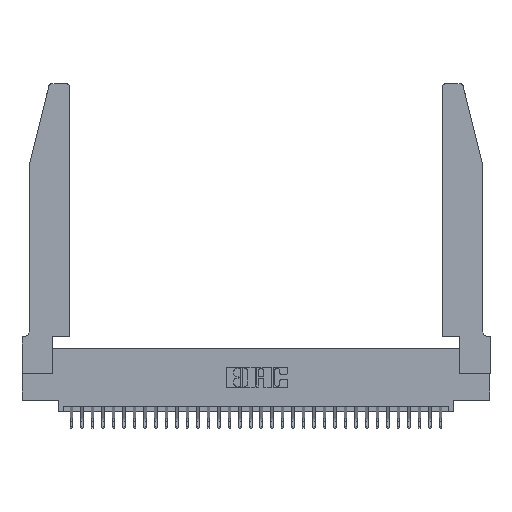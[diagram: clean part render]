
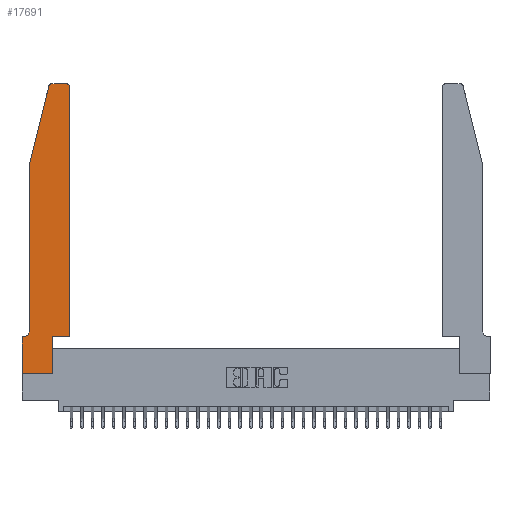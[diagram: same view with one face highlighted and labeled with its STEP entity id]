
A CAD part, top view. The second image highlights one B-rep face of the part: STEP entity #17691.
In plain terms, the highlighted planar face has unit normal (0, 0, 1).
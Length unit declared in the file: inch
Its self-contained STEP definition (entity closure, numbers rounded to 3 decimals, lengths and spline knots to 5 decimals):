
#825 = LINE ( 'NONE', #27042, #12400 ) ;
#1028 = ORIENTED_EDGE ( 'NONE', *, *, #27135, .T. ) ;
#1734 = CARTESIAN_POINT ( 'NONE',  ( 0., 0., 0.37 ) ) ;
#2498 = DIRECTION ( 'NONE',  ( 1., 0., 0. ) ) ;
#3057 = CARTESIAN_POINT ( 'NONE',  ( 0.0755, 2., 0.37 ) ) ;
#4718 = CARTESIAN_POINT ( 'NONE',  ( 0.284, 2.72, 0.37 ) ) ;
#4770 = CARTESIAN_POINT ( 'NONE',  ( 0.2865, 0.35, 0.37 ) ) ;
#4873 = CARTESIAN_POINT ( 'NONE',  ( 0.0755, 2., 0.37 ) ) ;
#4893 = VERTEX_POINT ( 'NONE', #19958 ) ;
#5174 = DIRECTION ( 'NONE',  ( -1., 0., 0. ) ) ;
#5564 = DIRECTION ( 'NONE',  ( 1., 0., 0. ) ) ;
#6221 = DIRECTION ( 'NONE',  ( 1., 0., 0. ) ) ;
#6347 = EDGE_CURVE ( 'NONE', #23144, #25207, #25120, .T. ) ;
#6566 = DIRECTION ( 'NONE',  ( 0., 0., -1. ) ) ;
#6980 = CARTESIAN_POINT ( 'NONE',  ( 0., 0., 0.37 ) ) ;
#7020 = VERTEX_POINT ( 'NONE', #27892 ) ;
#7575 = CIRCLE ( 'NONE', #29233, 0.03 ) ;
#7687 = EDGE_CURVE ( 'NONE', #19521, #7020, #26011, .T. ) ;
#7766 = CARTESIAN_POINT ( 'NONE',  ( 0.4505, 0.35, 0.37 ) ) ;
#8029 = PLANE ( 'NONE',  #14119 ) ;
#9557 = EDGE_CURVE ( 'NONE', #27238, #30307, #28830, .T. ) ;
#9586 = LINE ( 'NONE', #6980, #23934 ) ;
#9855 = CIRCLE ( 'NONE', #29030, 0.03 ) ;
#10363 = EDGE_LOOP ( 'NONE', ( #27302, #29611, #12300, #27228, #28320, #13306, #20744, #26653, #16598, #30921, #16795, #1028 ) ) ;
#11478 = CARTESIAN_POINT ( 'NONE',  ( 0., 0., 0.37 ) ) ;
#11808 = CARTESIAN_POINT ( 'NONE',  ( 0.0755, 0.42, 0.37 ) ) ;
#12132 = EDGE_CURVE ( 'NONE', #4893, #17674, #15429, .T. ) ;
#12299 = VERTEX_POINT ( 'NONE', #11808 ) ;
#12300 = ORIENTED_EDGE ( 'NONE', *, *, #31945, .T. ) ;
#12381 = VERTEX_POINT ( 'NONE', #29826 ) ;
#12400 = VECTOR ( 'NONE', #24616, 39.37008 ) ;
#13043 = LINE ( 'NONE', #7766, #18412 ) ;
#13194 = EDGE_CURVE ( 'NONE', #25207, #19521, #9586, .T. ) ;
#13252 = FACE_OUTER_BOUND ( 'NONE', #10363, .T. ) ;
#13306 = ORIENTED_EDGE ( 'NONE', *, *, #6347, .T. ) ;
#13780 = CARTESIAN_POINT ( 'NONE',  ( 0., 0.35, 0.37 ) ) ;
#13881 = VECTOR ( 'NONE', #18161, 39.37008 ) ;
#13905 = DIRECTION ( 'NONE',  ( 0., 0., 1. ) ) ;
#14119 = AXIS2_PLACEMENT_3D ( 'NONE', #13780, #13905, #6221 ) ;
#14196 = VERTEX_POINT ( 'NONE', #4873 ) ;
#14491 = CARTESIAN_POINT ( 'NONE',  ( 0.4505, 2.72, 0.37 ) ) ;
#14589 = CARTESIAN_POINT ( 'NONE',  ( 0., 0.35, 0.37 ) ) ;
#14876 = AXIS2_PLACEMENT_3D ( 'NONE', #22237, #6566, #19216 ) ;
#15040 = CARTESIAN_POINT ( 'NONE',  ( 0.0055, 0.35, 0.37 ) ) ;
#15410 = CARTESIAN_POINT ( 'NONE',  ( 0.284, 2.75, 0.37 ) ) ;
#15429 = LINE ( 'NONE', #28577, #28667 ) ;
#16598 = ORIENTED_EDGE ( 'NONE', *, *, #25202, .T. ) ;
#16795 = ORIENTED_EDGE ( 'NONE', *, *, #28310, .T. ) ;
#17674 = VERTEX_POINT ( 'NONE', #23502 ) ;
#17691 = ADVANCED_FACE ( 'NONE', ( #13252 ), #8029, .T. ) ;
#18132 = DIRECTION ( 'NONE',  ( 1., 0., 0. ) ) ;
#18161 = DIRECTION ( 'NONE',  ( -1., 0., 0. ) ) ;
#18412 = VECTOR ( 'NONE', #31124, 39.37008 ) ;
#18492 = VECTOR ( 'NONE', #5174, 39.37008 ) ;
#18809 = CARTESIAN_POINT ( 'NONE',  ( 0.4205, 2.72, 0.37 ) ) ;
#19210 = DIRECTION ( 'NONE',  ( 0., -1., 0. ) ) ;
#19216 = DIRECTION ( 'NONE',  ( -1., 0., 0. ) ) ;
#19521 = VERTEX_POINT ( 'NONE', #11478 ) ;
#19892 = DIRECTION ( 'NONE',  ( 0., 1., 0. ) ) ;
#19958 = CARTESIAN_POINT ( 'NONE',  ( 0.2865, 0.35, 0.37 ) ) ;
#20509 = CARTESIAN_POINT ( 'NONE',  ( 0.2605, 2.75, 0.37 ) ) ;
#20744 = ORIENTED_EDGE ( 'NONE', *, *, #13194, .T. ) ;
#20942 = EDGE_CURVE ( 'NONE', #30307, #12381, #7575, .T. ) ;
#21336 = CARTESIAN_POINT ( 'NONE',  ( 0.4205, 2.75, 0.37 ) ) ;
#21387 = EDGE_CURVE ( 'NONE', #12299, #23144, #31114, .T. ) ;
#21575 = DIRECTION ( 'NONE',  ( 0., 0., 1. ) ) ;
#21844 = VECTOR ( 'NONE', #25511, 39.37008 ) ;
#22237 = CARTESIAN_POINT ( 'NONE',  ( 0.0055, 0.42, 0.37 ) ) ;
#23144 = VERTEX_POINT ( 'NONE', #15040 ) ;
#23502 = CARTESIAN_POINT ( 'NONE',  ( 0.4505, 0.35, 0.37 ) ) ;
#23934 = VECTOR ( 'NONE', #31550, 39.37008 ) ;
#24616 = DIRECTION ( 'NONE',  ( -0.239, -0.971, 0. ) ) ;
#25120 = LINE ( 'NONE', #26395, #18492 ) ;
#25202 = EDGE_CURVE ( 'NONE', #7020, #4893, #30046, .T. ) ;
#25207 = VERTEX_POINT ( 'NONE', #14589 ) ;
#25511 = DIRECTION ( 'NONE',  ( 1., 0., 0. ) ) ;
#26011 = LINE ( 'NONE', #1734, #21844 ) ;
#26395 = CARTESIAN_POINT ( 'NONE',  ( 0.0755, 0.35, 0.37 ) ) ;
#26653 = ORIENTED_EDGE ( 'NONE', *, *, #7687, .T. ) ;
#27042 = CARTESIAN_POINT ( 'NONE',  ( 0.0755, 2., 0.37 ) ) ;
#27135 = EDGE_CURVE ( 'NONE', #29904, #27238, #9855, .T. ) ;
#27228 = ORIENTED_EDGE ( 'NONE', *, *, #27847, .T. ) ;
#27238 = VERTEX_POINT ( 'NONE', #21336 ) ;
#27302 = ORIENTED_EDGE ( 'NONE', *, *, #9557, .T. ) ;
#27847 = EDGE_CURVE ( 'NONE', #14196, #12299, #28385, .T. ) ;
#27892 = CARTESIAN_POINT ( 'NONE',  ( 0.2865, 0., 0.37 ) ) ;
#28310 = EDGE_CURVE ( 'NONE', #17674, #29904, #13043, .T. ) ;
#28320 = ORIENTED_EDGE ( 'NONE', *, *, #21387, .T. ) ;
#28385 = LINE ( 'NONE', #3057, #29582 ) ;
#28577 = CARTESIAN_POINT ( 'NONE',  ( 0.4505, 0.35, 0.37 ) ) ;
#28667 = VECTOR ( 'NONE', #18132, 39.37008 ) ;
#28830 = LINE ( 'NONE', #20509, #13881 ) ;
#29030 = AXIS2_PLACEMENT_3D ( 'NONE', #18809, #21575, #5564 ) ;
#29233 = AXIS2_PLACEMENT_3D ( 'NONE', #4718, #34125, #2498 ) ;
#29582 = VECTOR ( 'NONE', #19210, 39.37008 ) ;
#29611 = ORIENTED_EDGE ( 'NONE', *, *, #20942, .T. ) ;
#29826 = CARTESIAN_POINT ( 'NONE',  ( 0.25487, 2.72718, 0.37 ) ) ;
#29904 = VERTEX_POINT ( 'NONE', #14491 ) ;
#30046 = LINE ( 'NONE', #4770, #31712 ) ;
#30307 = VERTEX_POINT ( 'NONE', #15410 ) ;
#30921 = ORIENTED_EDGE ( 'NONE', *, *, #12132, .T. ) ;
#31114 = CIRCLE ( 'NONE', #14876, 0.07 ) ;
#31124 = DIRECTION ( 'NONE',  ( 0., 1., 0. ) ) ;
#31550 = DIRECTION ( 'NONE',  ( 0., -1., 0. ) ) ;
#31712 = VECTOR ( 'NONE', #19892, 39.37008 ) ;
#31945 = EDGE_CURVE ( 'NONE', #12381, #14196, #825, .T. ) ;
#34125 = DIRECTION ( 'NONE',  ( 0., 0., 1. ) ) ;
